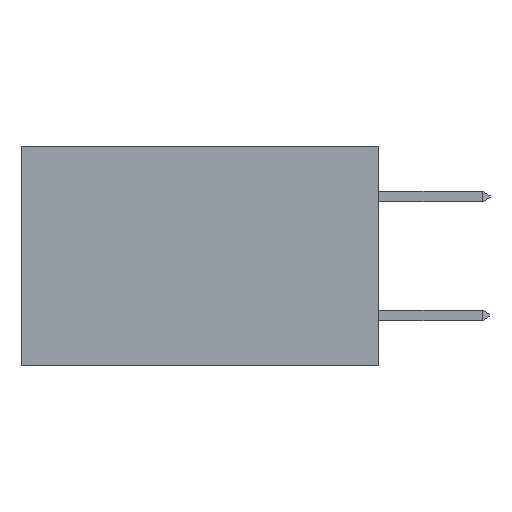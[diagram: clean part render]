
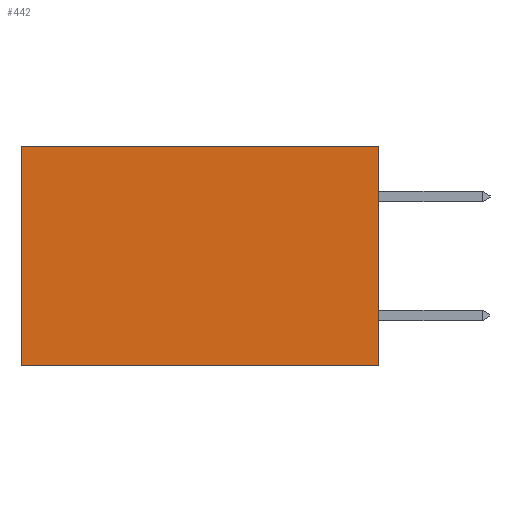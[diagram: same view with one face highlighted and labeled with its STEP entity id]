
A CAD part, left-side view. The second image highlights one B-rep face of the part: STEP entity #442.
In plain terms, the highlighted planar face has unit normal (-1, 0, 0).
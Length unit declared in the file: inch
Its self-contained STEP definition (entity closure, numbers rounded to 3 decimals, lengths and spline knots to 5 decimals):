
#442 = ADVANCED_FACE ( 'NONE', ( #6829 ), #11118, .F. ) ;
#1115 = DIRECTION ( 'NONE',  ( 0., 1., 0. ) ) ;
#1638 = DIRECTION ( 'NONE',  ( 1., 0., 0. ) ) ;
#2103 = LINE ( 'NONE', #12859, #5502 ) ;
#2678 = ORIENTED_EDGE ( 'NONE', *, *, #6059, .F. ) ;
#3599 = DIRECTION ( 'NONE',  ( 0., 1., 0. ) ) ;
#3672 = ORIENTED_EDGE ( 'NONE', *, *, #14411, .T. ) ;
#5104 = CARTESIAN_POINT ( 'NONE',  ( 0.298, 0., 0. ) ) ;
#5371 = DIRECTION ( 'NONE',  ( 0., 0., -1. ) ) ;
#5502 = VECTOR ( 'NONE', #1115, 39.37008 ) ;
#5892 = DIRECTION ( 'NONE',  ( 0., 0., -1. ) ) ;
#6059 = EDGE_CURVE ( 'NONE', #9734, #15768, #2103, .T. ) ;
#6829 = FACE_OUTER_BOUND ( 'NONE', #7609, .T. ) ;
#7609 = EDGE_LOOP ( 'NONE', ( #14235, #2678, #17708, #3672 ) ) ;
#8457 = LINE ( 'NONE', #15383, #15788 ) ;
#8994 = VECTOR ( 'NONE', #16108, 39.37008 ) ;
#9734 = VERTEX_POINT ( 'NONE', #13102 ) ;
#9795 = LINE ( 'NONE', #17141, #12773 ) ;
#11118 = PLANE ( 'NONE',  #12220 ) ;
#12220 = AXIS2_PLACEMENT_3D ( 'NONE', #5104, #1638, #5892 ) ;
#12320 = CARTESIAN_POINT ( 'NONE',  ( 0.298, 0., 0. ) ) ;
#12539 = CARTESIAN_POINT ( 'NONE',  ( 0.298, 0.6, -0.37 ) ) ;
#12632 = EDGE_CURVE ( 'NONE', #13048, #9734, #12896, .T. ) ;
#12773 = VECTOR ( 'NONE', #5371, 39.37008 ) ;
#12859 = CARTESIAN_POINT ( 'NONE',  ( 0.298, 0., -0.37 ) ) ;
#12896 = LINE ( 'NONE', #13161, #8994 ) ;
#13048 = VERTEX_POINT ( 'NONE', #12320 ) ;
#13102 = CARTESIAN_POINT ( 'NONE',  ( 0.298, 0., -0.37 ) ) ;
#13161 = CARTESIAN_POINT ( 'NONE',  ( 0.298, 0., 0. ) ) ;
#14235 = ORIENTED_EDGE ( 'NONE', *, *, #16184, .T. ) ;
#14411 = EDGE_CURVE ( 'NONE', #13048, #15125, #8457, .T. ) ;
#15125 = VERTEX_POINT ( 'NONE', #18458 ) ;
#15383 = CARTESIAN_POINT ( 'NONE',  ( 0.298, 0., 0. ) ) ;
#15768 = VERTEX_POINT ( 'NONE', #12539 ) ;
#15788 = VECTOR ( 'NONE', #3599, 39.37008 ) ;
#16108 = DIRECTION ( 'NONE',  ( 0., 0., -1. ) ) ;
#16184 = EDGE_CURVE ( 'NONE', #15125, #15768, #9795, .T. ) ;
#17141 = CARTESIAN_POINT ( 'NONE',  ( 0.298, 0.6, 0. ) ) ;
#17708 = ORIENTED_EDGE ( 'NONE', *, *, #12632, .F. ) ;
#18458 = CARTESIAN_POINT ( 'NONE',  ( 0.298, 0.6, 0. ) ) ;
